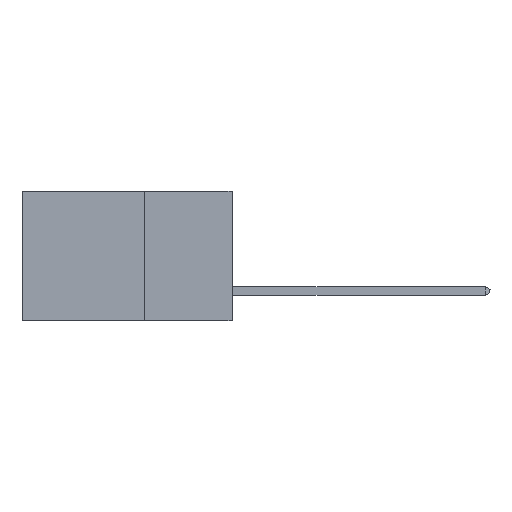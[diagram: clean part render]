
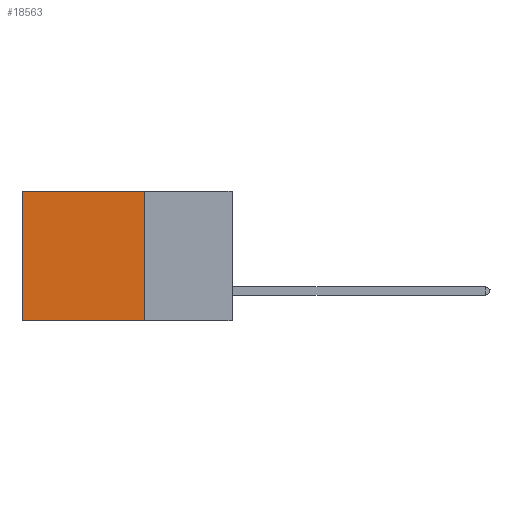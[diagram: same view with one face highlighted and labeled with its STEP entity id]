
A CAD part, left-side view. The second image highlights one B-rep face of the part: STEP entity #18563.
In plain terms, the highlighted planar face has unit normal (-1, 0, 0).
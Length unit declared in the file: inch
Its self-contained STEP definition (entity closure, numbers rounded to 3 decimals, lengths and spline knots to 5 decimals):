
#767 = VECTOR ( 'NONE', #33519, 39.37008 ) ;
#1689 = VECTOR ( 'NONE', #33908, 39.37008 ) ;
#2578 = CARTESIAN_POINT ( 'NONE',  ( 0.2875, 0.6, 0. ) ) ;
#2662 = DIRECTION ( 'NONE',  ( 0., 1., 0. ) ) ;
#5902 = VERTEX_POINT ( 'NONE', #2578 ) ;
#6236 = LINE ( 'NONE', #22029, #1689 ) ;
#7062 = AXIS2_PLACEMENT_3D ( 'NONE', #35390, #20797, #32792 ) ;
#8008 = CARTESIAN_POINT ( 'NONE',  ( 0.2875, 0.25, 0. ) ) ;
#9358 = DIRECTION ( 'NONE',  ( 0., 0., -1. ) ) ;
#10383 = LINE ( 'NONE', #36198, #767 ) ;
#10468 = VERTEX_POINT ( 'NONE', #8008 ) ;
#10827 = ORIENTED_EDGE ( 'NONE', *, *, #12243, .T. ) ;
#11790 = ORIENTED_EDGE ( 'NONE', *, *, #14112, .F. ) ;
#12243 = EDGE_CURVE ( 'NONE', #10468, #5902, #6236, .T. ) ;
#14112 = EDGE_CURVE ( 'NONE', #10468, #29189, #24290, .T. ) ;
#14281 = CARTESIAN_POINT ( 'NONE',  ( 0.2875, 0.25, -0.37 ) ) ;
#14721 = VECTOR ( 'NONE', #9358, 39.37008 ) ;
#14955 = PLANE ( 'NONE',  #7062 ) ;
#15946 = ORIENTED_EDGE ( 'NONE', *, *, #24781, .F. ) ;
#17165 = CARTESIAN_POINT ( 'NONE',  ( 0.2875, 0.6, -0.37 ) ) ;
#18563 = ADVANCED_FACE ( 'NONE', ( #23860 ), #14955, .F. ) ;
#19980 = VERTEX_POINT ( 'NONE', #17165 ) ;
#20797 = DIRECTION ( 'NONE',  ( 1., 0., 0. ) ) ;
#21549 = EDGE_CURVE ( 'NONE', #5902, #19980, #10383, .T. ) ;
#22029 = CARTESIAN_POINT ( 'NONE',  ( 0.2875, 0.25, 0. ) ) ;
#23860 = FACE_OUTER_BOUND ( 'NONE', #25542, .T. ) ;
#24290 = LINE ( 'NONE', #29480, #14721 ) ;
#24781 = EDGE_CURVE ( 'NONE', #29189, #19980, #34839, .T. ) ;
#25542 = EDGE_LOOP ( 'NONE', ( #31255, #15946, #11790, #10827 ) ) ;
#27047 = VECTOR ( 'NONE', #2662, 39.37008 ) ;
#29189 = VERTEX_POINT ( 'NONE', #32937 ) ;
#29480 = CARTESIAN_POINT ( 'NONE',  ( 0.2875, 0.25, 0. ) ) ;
#31255 = ORIENTED_EDGE ( 'NONE', *, *, #21549, .T. ) ;
#32792 = DIRECTION ( 'NONE',  ( 0., 0., -1. ) ) ;
#32937 = CARTESIAN_POINT ( 'NONE',  ( 0.2875, 0.25, -0.37 ) ) ;
#33519 = DIRECTION ( 'NONE',  ( 0., 0., -1. ) ) ;
#33908 = DIRECTION ( 'NONE',  ( 0., 1., 0. ) ) ;
#34839 = LINE ( 'NONE', #14281, #27047 ) ;
#35390 = CARTESIAN_POINT ( 'NONE',  ( 0.2875, 0.25, 0. ) ) ;
#36198 = CARTESIAN_POINT ( 'NONE',  ( 0.2875, 0.6, 0. ) ) ;
